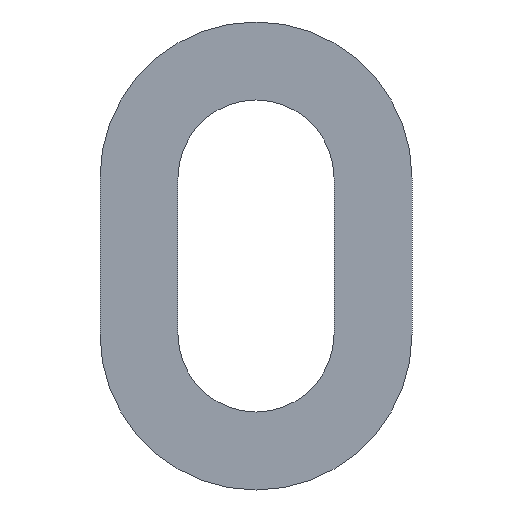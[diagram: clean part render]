
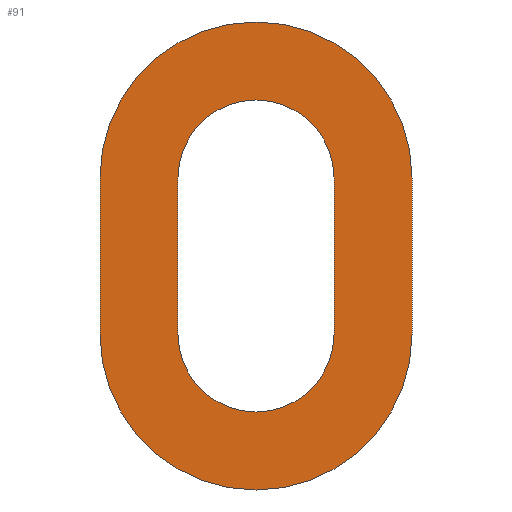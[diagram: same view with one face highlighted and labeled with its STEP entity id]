
A CAD part, front view. The second image highlights one B-rep face of the part: STEP entity #91.
In plain terms, the highlighted planar face has unit normal (0, -1, 0).
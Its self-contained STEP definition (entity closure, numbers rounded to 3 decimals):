
#3 = VERTEX_POINT ( 'NONE', #375 ) ;
#14 = AXIS2_PLACEMENT_3D ( 'NONE', #416, #129, #385 ) ;
#22 = ORIENTED_EDGE ( 'NONE', *, *, #176, .T. ) ;
#24 = VERTEX_POINT ( 'NONE', #417 ) ;
#32 = AXIS2_PLACEMENT_3D ( 'NONE', #321, #314, #318 ) ;
#34 = PLANE ( 'NONE',  #14 ) ;
#46 = AXIS2_PLACEMENT_3D ( 'NONE', #302, #295, #297 ) ;
#65 = AXIS2_PLACEMENT_3D ( 'NONE', #283, #288, #282 ) ;
#79 = AXIS2_PLACEMENT_3D ( 'NONE', #273, #270, #256 ) ;
#91 = ADVANCED_FACE ( 'NONE', ( #263, #245 ), #34, .F. ) ;
#119 = AXIS2_PLACEMENT_3D ( 'NONE', #266, #236, #240 ) ;
#129 = DIRECTION ( 'NONE',  ( 0., 1., 0. ) ) ;
#135 = DIRECTION ( 'NONE',  ( 0., 0., 1. ) ) ;
#137 = CARTESIAN_POINT ( 'NONE',  ( -2.5, 0., -5. ) ) ;
#140 = DIRECTION ( 'NONE',  ( 0., 1., 0. ) ) ;
#142 = CARTESIAN_POINT ( 'NONE',  ( 0., 0., -5. ) ) ;
#146 = EDGE_CURVE ( 'NONE', #415, #147, #211, .T. ) ;
#147 = VERTEX_POINT ( 'NONE', #365 ) ;
#155 = CARTESIAN_POINT ( 'NONE',  ( -5., 0., 0. ) ) ;
#156 = EDGE_CURVE ( 'NONE', #292, #415, #212, .T. ) ;
#161 = CARTESIAN_POINT ( 'NONE',  ( 2.5, 0., -5. ) ) ;
#166 = CIRCLE ( 'NONE', #177, 2.5 ) ;
#167 = EDGE_CURVE ( 'NONE', #311, #402, #215, .T. ) ;
#176 = EDGE_CURVE ( 'NONE', #147, #311, #222, .T. ) ;
#177 = AXIS2_PLACEMENT_3D ( 'NONE', #142, #140, #135 ) ;
#178 = CARTESIAN_POINT ( 'NONE',  ( -5., 0., -5. ) ) ;
#186 = CIRCLE ( 'NONE', #119, 5. ) ;
#187 = VECTOR ( 'NONE', #281, 1000. ) ;
#190 = EDGE_CURVE ( 'NONE', #3, #345, #204, .T. ) ;
#195 = CIRCLE ( 'NONE', #79, 5. ) ;
#198 = LINE ( 'NONE', #289, #187 ) ;
#200 = VECTOR ( 'NONE', #320, 1000. ) ;
#203 = CIRCLE ( 'NONE', #65, 5. ) ;
#204 = LINE ( 'NONE', #323, #200 ) ;
#205 = VECTOR ( 'NONE', #331, 1000. ) ;
#209 = VECTOR ( 'NONE', #328, 1000. ) ;
#211 = LINE ( 'NONE', #337, #209 ) ;
#212 = CIRCLE ( 'NONE', #32, 2.5 ) ;
#215 = LINE ( 'NONE', #326, #205 ) ;
#219 = CARTESIAN_POINT ( 'NONE',  ( 5., 0., -5. ) ) ;
#222 = CIRCLE ( 'NONE', #46, 2.5 ) ;
#226 = EDGE_CURVE ( 'NONE', #345, #24, #203, .T. ) ;
#236 = DIRECTION ( 'NONE',  ( 0., 1., 0. ) ) ;
#239 = EDGE_CURVE ( 'NONE', #391, #411, #198, .T. ) ;
#240 = DIRECTION ( 'NONE',  ( 0., 0., 1. ) ) ;
#242 = ORIENTED_EDGE ( 'NONE', *, *, #146, .T. ) ;
#245 = FACE_BOUND ( 'NONE', #303, .T. ) ;
#256 = DIRECTION ( 'NONE',  ( 0., 0., 1. ) ) ;
#258 = CARTESIAN_POINT ( 'NONE',  ( 2.5, 0., 0. ) ) ;
#260 = EDGE_CURVE ( 'NONE', #411, #3, #195, .T. ) ;
#263 = FACE_OUTER_BOUND ( 'NONE', #307, .T. ) ;
#266 = CARTESIAN_POINT ( 'NONE',  ( 0., 0., -5. ) ) ;
#270 = DIRECTION ( 'NONE',  ( 0., 1., 0. ) ) ;
#273 = CARTESIAN_POINT ( 'NONE',  ( 0., 0., 0. ) ) ;
#274 = CARTESIAN_POINT ( 'NONE',  ( 0., 0., -7.5 ) ) ;
#278 = ORIENTED_EDGE ( 'NONE', *, *, #167, .T. ) ;
#280 = EDGE_CURVE ( 'NONE', #24, #391, #186, .T. ) ;
#281 = DIRECTION ( 'NONE',  ( 0., 0., 1. ) ) ;
#282 = DIRECTION ( 'NONE',  ( 0., 0., 1. ) ) ;
#283 = CARTESIAN_POINT ( 'NONE',  ( 0., 0., -5. ) ) ;
#288 = DIRECTION ( 'NONE',  ( 0., 1., 0. ) ) ;
#289 = CARTESIAN_POINT ( 'NONE',  ( -5., 0., 0. ) ) ;
#292 = VERTEX_POINT ( 'NONE', #274 ) ;
#295 = DIRECTION ( 'NONE',  ( 0., 1., 0. ) ) ;
#297 = DIRECTION ( 'NONE',  ( 0., 0., 1. ) ) ;
#302 = CARTESIAN_POINT ( 'NONE',  ( 0., 0., 0. ) ) ;
#303 = EDGE_LOOP ( 'NONE', ( #22, #278, #407, #408, #242 ) ) ;
#307 = EDGE_LOOP ( 'NONE', ( #359, #360, #363, #364, #412 ) ) ;
#311 = VERTEX_POINT ( 'NONE', #258 ) ;
#314 = DIRECTION ( 'NONE',  ( 0., 1., 0. ) ) ;
#318 = DIRECTION ( 'NONE',  ( 0., 0., 1. ) ) ;
#320 = DIRECTION ( 'NONE',  ( 0., 0., -1. ) ) ;
#321 = CARTESIAN_POINT ( 'NONE',  ( 0., 0., -5. ) ) ;
#323 = CARTESIAN_POINT ( 'NONE',  ( 5., 0., 0. ) ) ;
#326 = CARTESIAN_POINT ( 'NONE',  ( 2.5, 0., 0. ) ) ;
#328 = DIRECTION ( 'NONE',  ( 0., 0., 1. ) ) ;
#331 = DIRECTION ( 'NONE',  ( 0., 0., -1. ) ) ;
#337 = CARTESIAN_POINT ( 'NONE',  ( -2.5, 0., 0. ) ) ;
#345 = VERTEX_POINT ( 'NONE', #219 ) ;
#359 = ORIENTED_EDGE ( 'NONE', *, *, #260, .F. ) ;
#360 = ORIENTED_EDGE ( 'NONE', *, *, #239, .F. ) ;
#363 = ORIENTED_EDGE ( 'NONE', *, *, #280, .F. ) ;
#364 = ORIENTED_EDGE ( 'NONE', *, *, #226, .F. ) ;
#365 = CARTESIAN_POINT ( 'NONE',  ( -2.5, 0., 0. ) ) ;
#375 = CARTESIAN_POINT ( 'NONE',  ( 5., 0., 0. ) ) ;
#385 = DIRECTION ( 'NONE',  ( 0., 0., 1. ) ) ;
#391 = VERTEX_POINT ( 'NONE', #178 ) ;
#402 = VERTEX_POINT ( 'NONE', #161 ) ;
#407 = ORIENTED_EDGE ( 'NONE', *, *, #410, .T. ) ;
#408 = ORIENTED_EDGE ( 'NONE', *, *, #156, .T. ) ;
#410 = EDGE_CURVE ( 'NONE', #402, #292, #166, .T. ) ;
#411 = VERTEX_POINT ( 'NONE', #155 ) ;
#412 = ORIENTED_EDGE ( 'NONE', *, *, #190, .F. ) ;
#415 = VERTEX_POINT ( 'NONE', #137 ) ;
#416 = CARTESIAN_POINT ( 'NONE',  ( 0., 0., 0. ) ) ;
#417 = CARTESIAN_POINT ( 'NONE',  ( 0., 0., -10. ) ) ;
